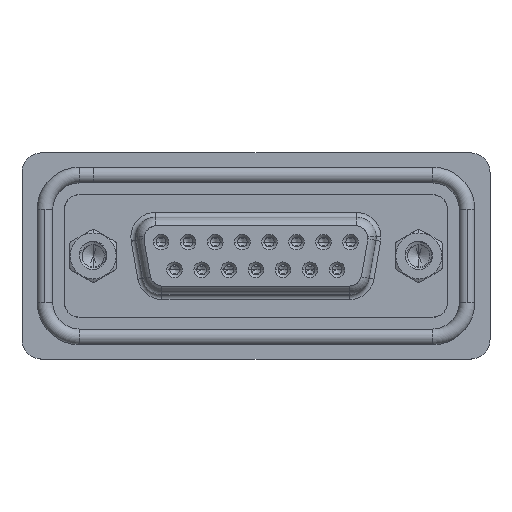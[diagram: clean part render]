
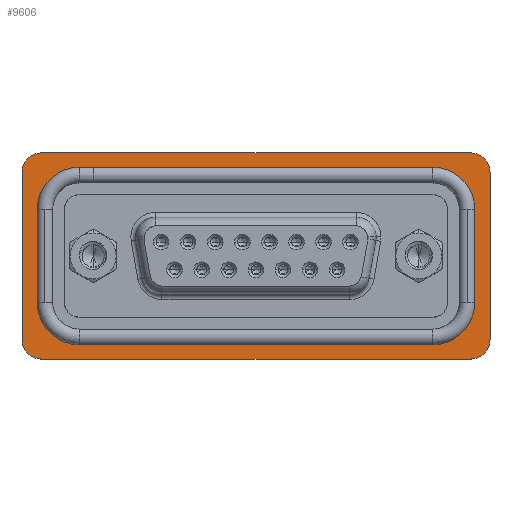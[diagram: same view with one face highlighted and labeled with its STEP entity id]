
A CAD part, top view. The second image highlights one B-rep face of the part: STEP entity #9606.
In plain terms, the highlighted planar face has unit normal (0, 0, 1).
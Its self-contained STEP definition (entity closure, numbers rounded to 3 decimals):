
#39 = CARTESIAN_POINT ( 'NONE',  ( -7.285, -8.55, 0.4 ) ) ;
#132 = LINE ( 'NONE', #23574, #21210 ) ;
#298 = VERTEX_POINT ( 'NONE', #11230 ) ;
#382 = VECTOR ( 'NONE', #3073, 1000. ) ;
#579 = DIRECTION ( 'NONE',  ( 0., 0., 1. ) ) ;
#809 = AXIS2_PLACEMENT_3D ( 'NONE', #18673, #4647, #6559 ) ;
#906 = AXIS2_PLACEMENT_3D ( 'NONE', #11179, #5490, #17341 ) ;
#984 = CARTESIAN_POINT ( 'NONE',  ( 38.605, 10.55, 0.4 ) ) ;
#1465 = DIRECTION ( 'NONE',  ( 0., 0., 1. ) ) ;
#1720 = CARTESIAN_POINT ( 'NONE',  ( 34.755, -4.775, 0.4 ) ) ;
#2045 = VERTEX_POINT ( 'NONE', #21224 ) ;
#2273 = CIRCLE ( 'NONE', #22407, 2. ) ;
#2655 = EDGE_CURVE ( 'NONE', #15501, #18839, #11377, .T. ) ;
#3073 = DIRECTION ( 'NONE',  ( 0., -1., 0. ) ) ;
#3316 = DIRECTION ( 'NONE',  ( 0., 0., 1. ) ) ;
#3322 = DIRECTION ( 'NONE',  ( 0., 0., 1. ) ) ;
#3383 = CARTESIAN_POINT ( 'NONE',  ( 38.605, -10.55, 0.4 ) ) ;
#3454 = EDGE_CURVE ( 'NONE', #10338, #10262, #18436, .T. ) ;
#3466 = ORIENTED_EDGE ( 'NONE', *, *, #7123, .F. ) ;
#3746 = DIRECTION ( 'NONE',  ( 1., 0., 0. ) ) ;
#3825 = FACE_OUTER_BOUND ( 'NONE', #24012, .T. ) ;
#4051 = EDGE_CURVE ( 'NONE', #9438, #298, #21299, .T. ) ;
#4057 = CARTESIAN_POINT ( 'NONE',  ( 39.055, -4.775, 0.4 ) ) ;
#4181 = AXIS2_PLACEMENT_3D ( 'NONE', #1720, #1465, #7492 ) ;
#4222 = LINE ( 'NONE', #984, #13216 ) ;
#4647 = DIRECTION ( 'NONE',  ( 0., 0., 1. ) ) ;
#4987 = CARTESIAN_POINT ( 'NONE',  ( -5.735, -4.775, 0.4 ) ) ;
#5100 = VERTEX_POINT ( 'NONE', #6350 ) ;
#5295 = AXIS2_PLACEMENT_3D ( 'NONE', #5491, #3322, #24921 ) ;
#5409 = ORIENTED_EDGE ( 'NONE', *, *, #5950, .T. ) ;
#5490 = DIRECTION ( 'NONE',  ( 0., 0., 1. ) ) ;
#5491 = CARTESIAN_POINT ( 'NONE',  ( -1.435, -4.775, 0.4 ) ) ;
#5548 = VERTEX_POINT ( 'NONE', #23824 ) ;
#5734 = FACE_BOUND ( 'NONE', #15573, .T. ) ;
#5808 = VECTOR ( 'NONE', #6637, 1000. ) ;
#5950 = EDGE_CURVE ( 'NONE', #22761, #10338, #19338, .T. ) ;
#6350 = CARTESIAN_POINT ( 'NONE',  ( 39.055, 4.775, 0.4 ) ) ;
#6394 = CARTESIAN_POINT ( 'NONE',  ( 38.605, 10.55, 0.4 ) ) ;
#6559 = DIRECTION ( 'NONE',  ( 1., 0., 0. ) ) ;
#6637 = DIRECTION ( 'NONE',  ( 0., -1., 0. ) ) ;
#7123 = EDGE_CURVE ( 'NONE', #2045, #17698, #19740, .T. ) ;
#7165 = CARTESIAN_POINT ( 'NONE',  ( -5.735, 4.775, 0.4 ) ) ;
#7372 = ORIENTED_EDGE ( 'NONE', *, *, #21837, .F. ) ;
#7492 = DIRECTION ( 'NONE',  ( 1., 0., 0. ) ) ;
#7980 = EDGE_CURVE ( 'NONE', #20322, #11096, #16069, .T. ) ;
#8269 = ORIENTED_EDGE ( 'NONE', *, *, #18232, .F. ) ;
#8398 = DIRECTION ( 'NONE',  ( 1., 0., 0. ) ) ;
#8633 = AXIS2_PLACEMENT_3D ( 'NONE', #14534, #8738, #22378 ) ;
#8674 = AXIS2_PLACEMENT_3D ( 'NONE', #21223, #15175, #19165 ) ;
#8729 = LINE ( 'NONE', #7165, #382 ) ;
#8738 = DIRECTION ( 'NONE',  ( 0., 0., 1. ) ) ;
#8896 = AXIS2_PLACEMENT_3D ( 'NONE', #20941, #3316, #11173 ) ;
#9438 = VERTEX_POINT ( 'NONE', #4987 ) ;
#9606 = ADVANCED_FACE ( 'NONE', ( #5734, #3825 ), #11682, .T. ) ;
#9883 = ORIENTED_EDGE ( 'NONE', *, *, #24596, .T. ) ;
#9933 = VECTOR ( 'NONE', #8398, 1000. ) ;
#10102 = VECTOR ( 'NONE', #15769, 1000. ) ;
#10262 = VERTEX_POINT ( 'NONE', #3383 ) ;
#10338 = VERTEX_POINT ( 'NONE', #15338 ) ;
#11096 = VERTEX_POINT ( 'NONE', #6394 ) ;
#11173 = DIRECTION ( 'NONE',  ( 1., 0., 0. ) ) ;
#11179 = CARTESIAN_POINT ( 'NONE',  ( 38.605, 8.55, 0.4 ) ) ;
#11202 = ORIENTED_EDGE ( 'NONE', *, *, #21228, .F. ) ;
#11230 = CARTESIAN_POINT ( 'NONE',  ( -1.435, -9.075, 0.4 ) ) ;
#11377 = CIRCLE ( 'NONE', #8896, 4.3 ) ;
#11562 = CARTESIAN_POINT ( 'NONE',  ( -5.285, 8.55, 0.4 ) ) ;
#11682 = PLANE ( 'NONE',  #906 ) ;
#12957 = DIRECTION ( 'NONE',  ( 0., 1., 0. ) ) ;
#13097 = CARTESIAN_POINT ( 'NONE',  ( -7.285, -8.55, 0.4 ) ) ;
#13216 = VECTOR ( 'NONE', #20937, 1000. ) ;
#13414 = CARTESIAN_POINT ( 'NONE',  ( -5.735, 4.775, 0.4 ) ) ;
#13795 = CARTESIAN_POINT ( 'NONE',  ( 40.605, 8.55, 0.4 ) ) ;
#13839 = AXIS2_PLACEMENT_3D ( 'NONE', #20406, #579, #22090 ) ;
#14120 = CARTESIAN_POINT ( 'NONE',  ( -7.285, 8.55, 0.4 ) ) ;
#14258 = VECTOR ( 'NONE', #3746, 1000. ) ;
#14487 = EDGE_CURVE ( 'NONE', #21355, #17323, #2273, .T. ) ;
#14492 = LINE ( 'NONE', #24521, #18441 ) ;
#14534 = CARTESIAN_POINT ( 'NONE',  ( -5.285, -8.55, 0.4 ) ) ;
#15158 = DIRECTION ( 'NONE',  ( 1., 0., 0. ) ) ;
#15175 = DIRECTION ( 'NONE',  ( 0., 0., 1. ) ) ;
#15338 = CARTESIAN_POINT ( 'NONE',  ( -5.285, -10.55, 0.4 ) ) ;
#15501 = VERTEX_POINT ( 'NONE', #22913 ) ;
#15573 = EDGE_LOOP ( 'NONE', ( #19957, #7372, #3466, #8269, #23402, #11202, #25238, #23045 ) ) ;
#15769 = DIRECTION ( 'NONE',  ( -1., 0., 0. ) ) ;
#16069 = CIRCLE ( 'NONE', #8674, 2. ) ;
#16193 = EDGE_CURVE ( 'NONE', #10262, #5548, #24922, .T. ) ;
#16347 = EDGE_CURVE ( 'NONE', #22664, #15501, #17694, .T. ) ;
#16457 = CIRCLE ( 'NONE', #809, 4.3 ) ;
#16875 = EDGE_CURVE ( 'NONE', #5548, #20322, #132, .T. ) ;
#17097 = DIRECTION ( 'NONE',  ( 0., 0., 1. ) ) ;
#17323 = VERTEX_POINT ( 'NONE', #14120 ) ;
#17341 = DIRECTION ( 'NONE',  ( 1., 0., 0. ) ) ;
#17542 = DIRECTION ( 'NONE',  ( 0., 1., 0. ) ) ;
#17694 = LINE ( 'NONE', #23846, #10102 ) ;
#17698 = VERTEX_POINT ( 'NONE', #4057 ) ;
#18053 = CARTESIAN_POINT ( 'NONE',  ( 38.605, -10.55, 0.4 ) ) ;
#18232 = EDGE_CURVE ( 'NONE', #298, #2045, #21498, .T. ) ;
#18348 = ORIENTED_EDGE ( 'NONE', *, *, #24540, .T. ) ;
#18436 = LINE ( 'NONE', #18053, #9933 ) ;
#18441 = VECTOR ( 'NONE', #12957, 1000. ) ;
#18673 = CARTESIAN_POINT ( 'NONE',  ( 34.755, 4.775, 0.4 ) ) ;
#18728 = ORIENTED_EDGE ( 'NONE', *, *, #7980, .T. ) ;
#18839 = VERTEX_POINT ( 'NONE', #13414 ) ;
#19150 = ORIENTED_EDGE ( 'NONE', *, *, #16193, .T. ) ;
#19165 = DIRECTION ( 'NONE',  ( 1., 0., 0. ) ) ;
#19338 = CIRCLE ( 'NONE', #8633, 2. ) ;
#19740 = CIRCLE ( 'NONE', #4181, 4.3 ) ;
#19957 = ORIENTED_EDGE ( 'NONE', *, *, #23145, .F. ) ;
#20322 = VERTEX_POINT ( 'NONE', #13795 ) ;
#20406 = CARTESIAN_POINT ( 'NONE',  ( 38.605, -8.55, 0.4 ) ) ;
#20705 = CARTESIAN_POINT ( 'NONE',  ( 34.755, 9.075, 0.4 ) ) ;
#20937 = DIRECTION ( 'NONE',  ( -1., 0., 0. ) ) ;
#20941 = CARTESIAN_POINT ( 'NONE',  ( -1.435, 4.775, 0.4 ) ) ;
#20975 = ORIENTED_EDGE ( 'NONE', *, *, #16875, .T. ) ;
#21210 = VECTOR ( 'NONE', #17542, 1000. ) ;
#21223 = CARTESIAN_POINT ( 'NONE',  ( 38.605, 8.55, 0.4 ) ) ;
#21224 = CARTESIAN_POINT ( 'NONE',  ( 34.755, -9.075, 0.4 ) ) ;
#21228 = EDGE_CURVE ( 'NONE', #18839, #9438, #8729, .T. ) ;
#21299 = CIRCLE ( 'NONE', #5295, 4.3 ) ;
#21326 = CARTESIAN_POINT ( 'NONE',  ( -5.285, 10.55, 0.4 ) ) ;
#21355 = VERTEX_POINT ( 'NONE', #21326 ) ;
#21366 = ORIENTED_EDGE ( 'NONE', *, *, #14487, .T. ) ;
#21498 = LINE ( 'NONE', #23554, #14258 ) ;
#21837 = EDGE_CURVE ( 'NONE', #17698, #5100, #14492, .T. ) ;
#22090 = DIRECTION ( 'NONE',  ( 1., 0., 0. ) ) ;
#22378 = DIRECTION ( 'NONE',  ( -1., 0., 0. ) ) ;
#22407 = AXIS2_PLACEMENT_3D ( 'NONE', #11562, #17097, #15158 ) ;
#22664 = VERTEX_POINT ( 'NONE', #20705 ) ;
#22761 = VERTEX_POINT ( 'NONE', #39 ) ;
#22872 = LINE ( 'NONE', #13097, #5808 ) ;
#22913 = CARTESIAN_POINT ( 'NONE',  ( -1.435, 9.075, 0.4 ) ) ;
#23045 = ORIENTED_EDGE ( 'NONE', *, *, #16347, .F. ) ;
#23145 = EDGE_CURVE ( 'NONE', #5100, #22664, #16457, .T. ) ;
#23402 = ORIENTED_EDGE ( 'NONE', *, *, #4051, .F. ) ;
#23554 = CARTESIAN_POINT ( 'NONE',  ( -1.435, -9.075, 0.4 ) ) ;
#23574 = CARTESIAN_POINT ( 'NONE',  ( 40.605, -8.55, 0.4 ) ) ;
#23824 = CARTESIAN_POINT ( 'NONE',  ( 40.605, -8.55, 0.4 ) ) ;
#23846 = CARTESIAN_POINT ( 'NONE',  ( 34.755, 9.075, 0.4 ) ) ;
#24012 = EDGE_LOOP ( 'NONE', ( #18728, #18348, #21366, #9883, #5409, #25383, #19150, #20975 ) ) ;
#24521 = CARTESIAN_POINT ( 'NONE',  ( 39.055, -4.775, 0.4 ) ) ;
#24540 = EDGE_CURVE ( 'NONE', #11096, #21355, #4222, .T. ) ;
#24596 = EDGE_CURVE ( 'NONE', #17323, #22761, #22872, .T. ) ;
#24921 = DIRECTION ( 'NONE',  ( 1., 0., 0. ) ) ;
#24922 = CIRCLE ( 'NONE', #13839, 2. ) ;
#25238 = ORIENTED_EDGE ( 'NONE', *, *, #2655, .F. ) ;
#25383 = ORIENTED_EDGE ( 'NONE', *, *, #3454, .T. ) ;
